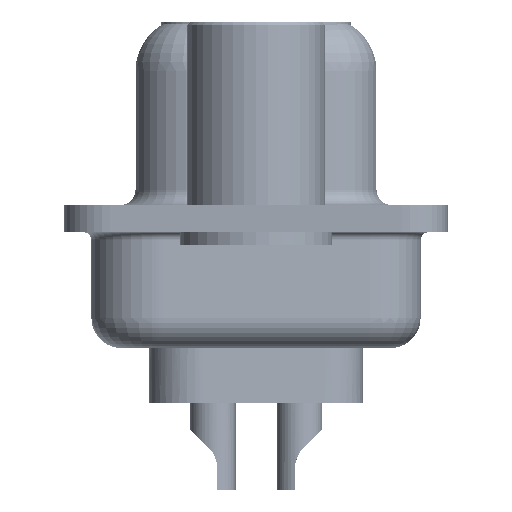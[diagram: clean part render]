
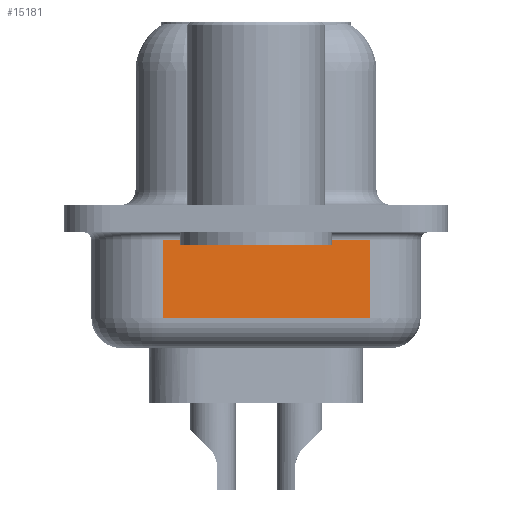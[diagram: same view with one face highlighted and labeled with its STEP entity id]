
A CAD part, left-side view. The second image highlights one B-rep face of the part: STEP entity #15181.
In plain terms, the highlighted planar face has unit normal (-0.985, -0.174, 0).
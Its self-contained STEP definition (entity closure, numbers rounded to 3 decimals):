
#389 = FACE_OUTER_BOUND ( 'NONE', #8319, .T. ) ;
#766 = VECTOR ( 'NONE', #13168, 1000. ) ;
#952 = ORIENTED_EDGE ( 'NONE', *, *, #18488, .F. ) ;
#1904 = ORIENTED_EDGE ( 'NONE', *, *, #16539, .T. ) ;
#2253 = CARTESIAN_POINT ( 'NONE',  ( 2.88, 3.053, -0.7 ) ) ;
#2346 = CARTESIAN_POINT ( 'NONE',  ( 4.079, -3.747, -3.25 ) ) ;
#2743 = PLANE ( 'NONE',  #14321 ) ;
#3537 = CARTESIAN_POINT ( 'NONE',  ( 2.88, 3.053, -3.25 ) ) ;
#4030 = CARTESIAN_POINT ( 'NONE',  ( 4.079, -3.747, -4.25 ) ) ;
#4075 = LINE ( 'NONE', #11152, #16904 ) ;
#4838 = LINE ( 'NONE', #7049, #5579 ) ;
#5579 = VECTOR ( 'NONE', #7351, 1000. ) ;
#5726 = VECTOR ( 'NONE', #25727, 1000. ) ;
#6133 = DIRECTION ( 'NONE',  ( 0., 0., 1. ) ) ;
#7049 = CARTESIAN_POINT ( 'NONE',  ( 2.88, 3.053, -0.7 ) ) ;
#7351 = DIRECTION ( 'NONE',  ( -0.174, 0.985, 0. ) ) ;
#8319 = EDGE_LOOP ( 'NONE', ( #952, #1904, #11097, #10633 ) ) ;
#10633 = ORIENTED_EDGE ( 'NONE', *, *, #24674, .T. ) ;
#11097 = ORIENTED_EDGE ( 'NONE', *, *, #14526, .T. ) ;
#11152 = CARTESIAN_POINT ( 'NONE',  ( 2.88, 3.053, -4.25 ) ) ;
#11273 = VERTEX_POINT ( 'NONE', #2346 ) ;
#12473 = VERTEX_POINT ( 'NONE', #16255 ) ;
#12771 = LINE ( 'NONE', #4030, #5726 ) ;
#13168 = DIRECTION ( 'NONE',  ( 0.174, -0.985, 0. ) ) ;
#13838 = VERTEX_POINT ( 'NONE', #2253 ) ;
#14321 = AXIS2_PLACEMENT_3D ( 'NONE', #15176, #27266, #22050 ) ;
#14526 = EDGE_CURVE ( 'NONE', #11273, #26547, #12771, .T. ) ;
#15176 = CARTESIAN_POINT ( 'NONE',  ( 2.88, 3.053, -4.25 ) ) ;
#15181 = ADVANCED_FACE ( 'NONE', ( #389 ), #2743, .F. ) ;
#15527 = LINE ( 'NONE', #3537, #766 ) ;
#16255 = CARTESIAN_POINT ( 'NONE',  ( 2.88, 3.053, -3.25 ) ) ;
#16539 = EDGE_CURVE ( 'NONE', #12473, #11273, #15527, .T. ) ;
#16904 = VECTOR ( 'NONE', #6133, 1000. ) ;
#18488 = EDGE_CURVE ( 'NONE', #12473, #13838, #4075, .T. ) ;
#22050 = DIRECTION ( 'NONE',  ( -0.174, 0.985, 0. ) ) ;
#24674 = EDGE_CURVE ( 'NONE', #26547, #13838, #4838, .T. ) ;
#25727 = DIRECTION ( 'NONE',  ( 0., 0., 1. ) ) ;
#26547 = VERTEX_POINT ( 'NONE', #29346 ) ;
#27266 = DIRECTION ( 'NONE',  ( 0.985, 0.174, 0. ) ) ;
#29346 = CARTESIAN_POINT ( 'NONE',  ( 4.079, -3.747, -0.7 ) ) ;
